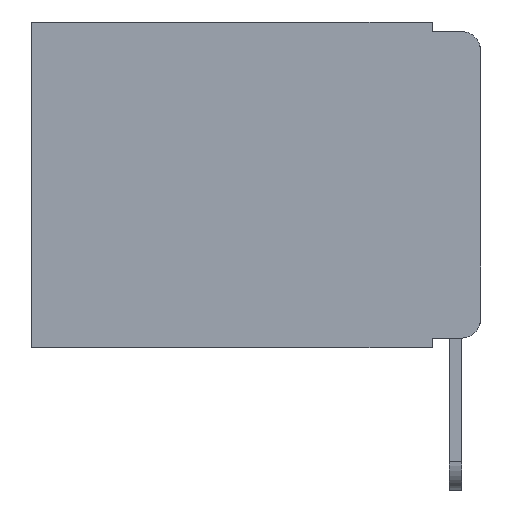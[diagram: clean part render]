
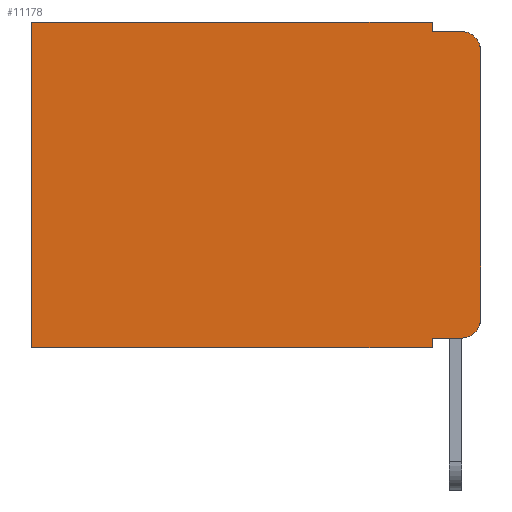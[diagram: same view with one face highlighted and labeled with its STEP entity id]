
A CAD part, left-side view. The second image highlights one B-rep face of the part: STEP entity #11178.
In plain terms, the highlighted planar face has unit normal (-1, 0, 0).
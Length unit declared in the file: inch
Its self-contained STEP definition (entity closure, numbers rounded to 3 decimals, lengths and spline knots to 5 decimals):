
#79 = ORIENTED_EDGE ( 'NONE', *, *, #6717, .F. ) ;
#212 = VERTEX_POINT ( 'NONE', #7387 ) ;
#219 = CARTESIAN_POINT ( 'NONE',  ( 0.298, 0., -0.343 ) ) ;
#380 = EDGE_CURVE ( 'NONE', #7970, #7502, #898, .T. ) ;
#627 = CARTESIAN_POINT ( 'NONE',  ( 0.298, 0.051, -0.01 ) ) ;
#766 = EDGE_CURVE ( 'NONE', #7970, #1764, #7511, .T. ) ;
#898 = LINE ( 'NONE', #11765, #3445 ) ;
#929 = VECTOR ( 'NONE', #5138, 39.37008 ) ;
#1185 = DIRECTION ( 'NONE',  ( 0., 0., -1. ) ) ;
#1210 = ORIENTED_EDGE ( 'NONE', *, *, #12141, .T. ) ;
#1230 = DIRECTION ( 'NONE',  ( 0., -1., 0. ) ) ;
#1246 = ORIENTED_EDGE ( 'NONE', *, *, #380, .F. ) ;
#1314 = CARTESIAN_POINT ( 'NONE',  ( 0.298, 0.051, 0. ) ) ;
#1574 = ORIENTED_EDGE ( 'NONE', *, *, #6273, .T. ) ;
#1715 = EDGE_CURVE ( 'NONE', #9899, #212, #8004, .T. ) ;
#1764 = VERTEX_POINT ( 'NONE', #9650 ) ;
#1769 = LINE ( 'NONE', #219, #11358 ) ;
#1981 = CARTESIAN_POINT ( 'NONE',  ( 0.298, 0.051, -0.333 ) ) ;
#2052 = CARTESIAN_POINT ( 'NONE',  ( 0.298, 0., 0. ) ) ;
#2061 = VERTEX_POINT ( 'NONE', #11085 ) ;
#2264 = EDGE_CURVE ( 'NONE', #1764, #4181, #6904, .T. ) ;
#2486 = CARTESIAN_POINT ( 'NONE',  ( 0.298, 0.473, 0. ) ) ;
#2504 = DIRECTION ( 'NONE',  ( 0., 1., 0. ) ) ;
#2510 = EDGE_LOOP ( 'NONE', ( #8118, #1210, #2559, #79, #1574, #2924, #4328, #1246, #3072, #3342 ) ) ;
#2559 = ORIENTED_EDGE ( 'NONE', *, *, #1715, .F. ) ;
#2924 = ORIENTED_EDGE ( 'NONE', *, *, #6618, .T. ) ;
#3072 = ORIENTED_EDGE ( 'NONE', *, *, #766, .T. ) ;
#3342 = ORIENTED_EDGE ( 'NONE', *, *, #2264, .T. ) ;
#3445 = VECTOR ( 'NONE', #6702, 39.37008 ) ;
#3637 = VECTOR ( 'NONE', #7383, 39.37008 ) ;
#3809 = LINE ( 'NONE', #2052, #929 ) ;
#3848 = VERTEX_POINT ( 'NONE', #1314 ) ;
#3896 = DIRECTION ( 'NONE',  ( 0., 0., -1. ) ) ;
#3977 = LINE ( 'NONE', #2486, #3637 ) ;
#4097 = VERTEX_POINT ( 'NONE', #11078 ) ;
#4181 = VERTEX_POINT ( 'NONE', #5010 ) ;
#4214 = LINE ( 'NONE', #10255, #8585 ) ;
#4328 = ORIENTED_EDGE ( 'NONE', *, *, #11009, .F. ) ;
#4939 = DIRECTION ( 'NONE',  ( 0., -1., 0. ) ) ;
#4989 = FACE_OUTER_BOUND ( 'NONE', #2510, .T. ) ;
#5010 = CARTESIAN_POINT ( 'NONE',  ( 0.298, 0., -0.313 ) ) ;
#5060 = DIRECTION ( 'NONE',  ( 0., 0., -1. ) ) ;
#5138 = DIRECTION ( 'NONE',  ( 0., 1., 0. ) ) ;
#5220 = AXIS2_PLACEMENT_3D ( 'NONE', #9372, #7212, #1185 ) ;
#5567 = VECTOR ( 'NONE', #4939, 39.37008 ) ;
#5636 = CARTESIAN_POINT ( 'NONE',  ( 0.298, 0.051, 0. ) ) ;
#5651 = VECTOR ( 'NONE', #7499, 39.37008 ) ;
#5707 = CIRCLE ( 'NONE', #5220, 0.02 ) ;
#6273 = EDGE_CURVE ( 'NONE', #3848, #4097, #3809, .T. ) ;
#6618 = EDGE_CURVE ( 'NONE', #4097, #7110, #3977, .T. ) ;
#6702 = DIRECTION ( 'NONE',  ( 0., 0., -1. ) ) ;
#6717 = EDGE_CURVE ( 'NONE', #3848, #9899, #10376, .T. ) ;
#6786 = AXIS2_PLACEMENT_3D ( 'NONE', #10232, #9448, #3896 ) ;
#6904 = CIRCLE ( 'NONE', #11590, 0.02 ) ;
#7110 = VERTEX_POINT ( 'NONE', #11566 ) ;
#7175 = CARTESIAN_POINT ( 'NONE',  ( 0.298, 0.051, -0.343 ) ) ;
#7212 = DIRECTION ( 'NONE',  ( -1., 0., 0. ) ) ;
#7383 = DIRECTION ( 'NONE',  ( 0., 0., -1. ) ) ;
#7387 = CARTESIAN_POINT ( 'NONE',  ( 0.298, 0.02, -0.01 ) ) ;
#7499 = DIRECTION ( 'NONE',  ( 0., 0., -1. ) ) ;
#7502 = VERTEX_POINT ( 'NONE', #7175 ) ;
#7511 = LINE ( 'NONE', #7801, #10090 ) ;
#7801 = CARTESIAN_POINT ( 'NONE',  ( 0.298, 0.051, -0.333 ) ) ;
#7970 = VERTEX_POINT ( 'NONE', #1981 ) ;
#8004 = LINE ( 'NONE', #627, #5567 ) ;
#8118 = ORIENTED_EDGE ( 'NONE', *, *, #11928, .F. ) ;
#8585 = VECTOR ( 'NONE', #8596, 39.37008 ) ;
#8596 = DIRECTION ( 'NONE',  ( 0., 0., -1. ) ) ;
#9372 = CARTESIAN_POINT ( 'NONE',  ( 0.298, 0.02, -0.03 ) ) ;
#9448 = DIRECTION ( 'NONE',  ( 1., 0., 0. ) ) ;
#9496 = CARTESIAN_POINT ( 'NONE',  ( 0.298, 0.051, -0.01 ) ) ;
#9650 = CARTESIAN_POINT ( 'NONE',  ( 0.298, 0.02, -0.333 ) ) ;
#9899 = VERTEX_POINT ( 'NONE', #9496 ) ;
#10029 = DIRECTION ( 'NONE',  ( -1., 0., 0. ) ) ;
#10090 = VECTOR ( 'NONE', #1230, 39.37008 ) ;
#10232 = CARTESIAN_POINT ( 'NONE',  ( 0.298, 0., 0. ) ) ;
#10255 = CARTESIAN_POINT ( 'NONE',  ( 0.298, 0., 0. ) ) ;
#10376 = LINE ( 'NONE', #5636, #5651 ) ;
#10963 = CARTESIAN_POINT ( 'NONE',  ( 0.298, 0.02, -0.313 ) ) ;
#11009 = EDGE_CURVE ( 'NONE', #7502, #7110, #1769, .T. ) ;
#11044 = PLANE ( 'NONE',  #6786 ) ;
#11078 = CARTESIAN_POINT ( 'NONE',  ( 0.298, 0.473, 0. ) ) ;
#11085 = CARTESIAN_POINT ( 'NONE',  ( 0.298, 0., -0.03 ) ) ;
#11178 = ADVANCED_FACE ( 'NONE', ( #4989 ), #11044, .F. ) ;
#11358 = VECTOR ( 'NONE', #2504, 39.37008 ) ;
#11566 = CARTESIAN_POINT ( 'NONE',  ( 0.298, 0.473, -0.343 ) ) ;
#11590 = AXIS2_PLACEMENT_3D ( 'NONE', #10963, #10029, #5060 ) ;
#11765 = CARTESIAN_POINT ( 'NONE',  ( 0.298, 0.051, 0. ) ) ;
#11928 = EDGE_CURVE ( 'NONE', #2061, #4181, #4214, .T. ) ;
#12141 = EDGE_CURVE ( 'NONE', #2061, #212, #5707, .T. ) ;
